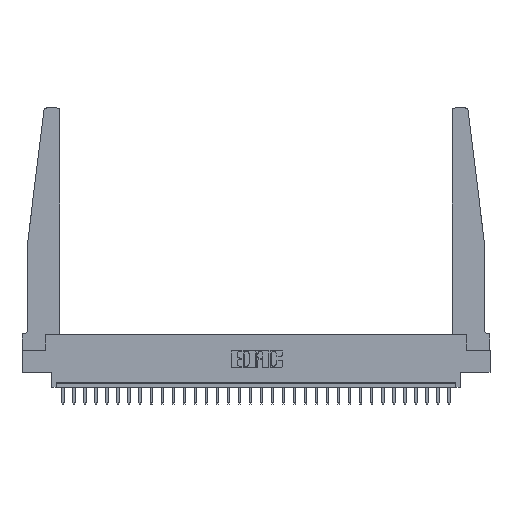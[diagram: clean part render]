
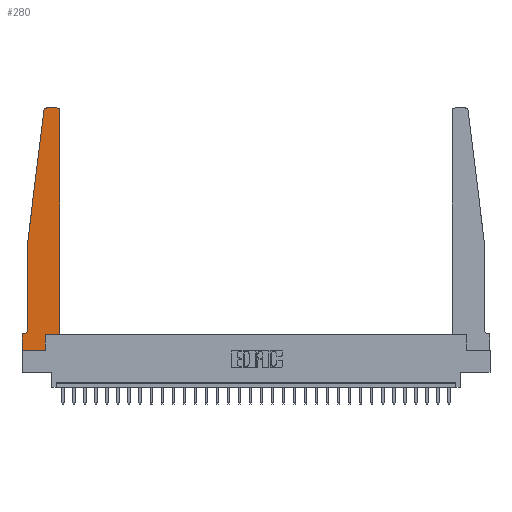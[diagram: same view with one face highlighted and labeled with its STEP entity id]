
A CAD part, top view. The second image highlights one B-rep face of the part: STEP entity #280.
In plain terms, the highlighted planar face has unit normal (0, 0, 1).
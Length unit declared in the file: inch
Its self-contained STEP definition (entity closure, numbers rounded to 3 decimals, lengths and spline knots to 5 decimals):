
#280 = ADVANCED_FACE ( 'NONE', ( #17258 ), #15068, .T. ) ;
#375 = CIRCLE ( 'NONE', #2223, 0.05 ) ;
#410 = VECTOR ( 'NONE', #20991, 39.37008 ) ;
#855 = CARTESIAN_POINT ( 'NONE',  ( 0.2605, 0.18, 0.37 ) ) ;
#1025 = DIRECTION ( 'NONE',  ( -1., 0., 0. ) ) ;
#1101 = EDGE_CURVE ( 'NONE', #24058, #24308, #16707, .T. ) ;
#1315 = CARTESIAN_POINT ( 'NONE',  ( 0., 0., 0.37 ) ) ;
#1605 = CARTESIAN_POINT ( 'NONE',  ( 0.395, 2.75, 0.37 ) ) ;
#1904 = CARTESIAN_POINT ( 'NONE',  ( 0., 0.1875, 0.37 ) ) ;
#2104 = EDGE_LOOP ( 'NONE', ( #17373, #17752, #11863, #24557, #27052, #9151, #11332, #17561, #2962, #5431, #9153, #21546 ) ) ;
#2171 = DIRECTION ( 'NONE',  ( 0., 0., 1. ) ) ;
#2223 = AXIS2_PLACEMENT_3D ( 'NONE', #21859, #21561, #15331 ) ;
#2415 = EDGE_CURVE ( 'NONE', #8377, #7073, #9239, .T. ) ;
#2419 = CARTESIAN_POINT ( 'NONE',  ( 0.2605, 0.18, 0.37 ) ) ;
#2713 = CARTESIAN_POINT ( 'NONE',  ( 0., 0., 0.37 ) ) ;
#2962 = ORIENTED_EDGE ( 'NONE', *, *, #15826, .T. ) ;
#3213 = VECTOR ( 'NONE', #13120, 39.37008 ) ;
#3463 = LINE ( 'NONE', #855, #19608 ) ;
#3505 = CARTESIAN_POINT ( 'NONE',  ( 0.2605, 0., 0.37 ) ) ;
#4042 = EDGE_CURVE ( 'NONE', #24308, #20543, #25350, .T. ) ;
#4122 = VERTEX_POINT ( 'NONE', #23754 ) ;
#4475 = LINE ( 'NONE', #24180, #3213 ) ;
#5311 = DIRECTION ( 'NONE',  ( 0., 1., 0. ) ) ;
#5431 = ORIENTED_EDGE ( 'NONE', *, *, #23795, .T. ) ;
#5452 = VECTOR ( 'NONE', #21392, 39.37008 ) ;
#5654 = AXIS2_PLACEMENT_3D ( 'NONE', #1904, #23916, #10833 ) ;
#5894 = EDGE_CURVE ( 'NONE', #11789, #4122, #375, .T. ) ;
#6534 = LINE ( 'NONE', #15383, #9674 ) ;
#7073 = VERTEX_POINT ( 'NONE', #15373 ) ;
#7841 = CARTESIAN_POINT ( 'NONE',  ( 0.425, 0.18, 0.37 ) ) ;
#8126 = DIRECTION ( 'NONE',  ( 1., 0., 0. ) ) ;
#8315 = VECTOR ( 'NONE', #11732, 39.37008 ) ;
#8377 = VERTEX_POINT ( 'NONE', #17723 ) ;
#8596 = VECTOR ( 'NONE', #1025, 39.37008 ) ;
#9109 = EDGE_CURVE ( 'NONE', #25172, #11789, #6534, .T. ) ;
#9151 = ORIENTED_EDGE ( 'NONE', *, *, #18477, .T. ) ;
#9153 = ORIENTED_EDGE ( 'NONE', *, *, #9848, .T. ) ;
#9239 = LINE ( 'NONE', #2713, #23352 ) ;
#9674 = VECTOR ( 'NONE', #24224, 39.37008 ) ;
#9848 = EDGE_CURVE ( 'NONE', #23096, #24058, #13945, .T. ) ;
#10488 = VERTEX_POINT ( 'NONE', #12768 ) ;
#10833 = DIRECTION ( 'NONE',  ( 1., 0., 0. ) ) ;
#11331 = DIRECTION ( 'NONE',  ( 0., 0., 1. ) ) ;
#11332 = ORIENTED_EDGE ( 'NONE', *, *, #2415, .T. ) ;
#11732 = DIRECTION ( 'NONE',  ( 0., 1., 0. ) ) ;
#11789 = VERTEX_POINT ( 'NONE', #21066 ) ;
#11863 = ORIENTED_EDGE ( 'NONE', *, *, #24391, .T. ) ;
#11987 = LINE ( 'NONE', #20853, #18716 ) ;
#12255 = CARTESIAN_POINT ( 'NONE',  ( 0.25, 2.75, 0.37 ) ) ;
#12768 = CARTESIAN_POINT ( 'NONE',  ( 0.24675, 2.72367, 0.37 ) ) ;
#13120 = DIRECTION ( 'NONE',  ( -0.122, -0.992, 0. ) ) ;
#13945 = LINE ( 'NONE', #25256, #8315 ) ;
#14062 = VERTEX_POINT ( 'NONE', #3505 ) ;
#14251 = CARTESIAN_POINT ( 'NONE',  ( 0.425, 2.72, 0.37 ) ) ;
#14354 = AXIS2_PLACEMENT_3D ( 'NONE', #19769, #11331, #17905 ) ;
#15068 = PLANE ( 'NONE',  #5654 ) ;
#15331 = DIRECTION ( 'NONE',  ( -1., 0., 0. ) ) ;
#15373 = CARTESIAN_POINT ( 'NONE',  ( 0., 0., 0.37 ) ) ;
#15383 = CARTESIAN_POINT ( 'NONE',  ( 0.065, 1.25, 0.37 ) ) ;
#15744 = CIRCLE ( 'NONE', #14354, 0.03 ) ;
#15826 = EDGE_CURVE ( 'NONE', #14062, #19433, #3463, .T. ) ;
#16707 = CIRCLE ( 'NONE', #27169, 0.03 ) ;
#17121 = CARTESIAN_POINT ( 'NONE',  ( 0.395, 2.72, 0.37 ) ) ;
#17197 = LINE ( 'NONE', #27630, #5452 ) ;
#17258 = FACE_OUTER_BOUND ( 'NONE', #2104, .T. ) ;
#17373 = ORIENTED_EDGE ( 'NONE', *, *, #4042, .T. ) ;
#17403 = DIRECTION ( 'NONE',  ( 0., -1., 0. ) ) ;
#17561 = ORIENTED_EDGE ( 'NONE', *, *, #22574, .T. ) ;
#17723 = CARTESIAN_POINT ( 'NONE',  ( 0., 0.1875, 0.37 ) ) ;
#17752 = ORIENTED_EDGE ( 'NONE', *, *, #26109, .T. ) ;
#17905 = DIRECTION ( 'NONE',  ( 1., 0., 0. ) ) ;
#18477 = EDGE_CURVE ( 'NONE', #4122, #8377, #11987, .T. ) ;
#18716 = VECTOR ( 'NONE', #25371, 39.37008 ) ;
#18942 = CARTESIAN_POINT ( 'NONE',  ( 0.27653, 2.75, 0.37 ) ) ;
#19433 = VERTEX_POINT ( 'NONE', #2419 ) ;
#19608 = VECTOR ( 'NONE', #5311, 39.37008 ) ;
#19769 = CARTESIAN_POINT ( 'NONE',  ( 0.27653, 2.72, 0.37 ) ) ;
#20543 = VERTEX_POINT ( 'NONE', #18942 ) ;
#20853 = CARTESIAN_POINT ( 'NONE',  ( 0.065, 0.1875, 0.37 ) ) ;
#20991 = DIRECTION ( 'NONE',  ( 1., 0., 0. ) ) ;
#21066 = CARTESIAN_POINT ( 'NONE',  ( 0.065, 0.2375, 0.37 ) ) ;
#21392 = DIRECTION ( 'NONE',  ( 1., 0., 0. ) ) ;
#21546 = ORIENTED_EDGE ( 'NONE', *, *, #1101, .T. ) ;
#21561 = DIRECTION ( 'NONE',  ( 0., 0., -1. ) ) ;
#21859 = CARTESIAN_POINT ( 'NONE',  ( 0.015, 0.2375, 0.37 ) ) ;
#21888 = CARTESIAN_POINT ( 'NONE',  ( 0.065, 1.25, 0.37 ) ) ;
#22574 = EDGE_CURVE ( 'NONE', #7073, #14062, #27821, .T. ) ;
#23096 = VERTEX_POINT ( 'NONE', #7841 ) ;
#23352 = VECTOR ( 'NONE', #17403, 39.37008 ) ;
#23754 = CARTESIAN_POINT ( 'NONE',  ( 0.015, 0.1875, 0.37 ) ) ;
#23795 = EDGE_CURVE ( 'NONE', #19433, #23096, #17197, .T. ) ;
#23916 = DIRECTION ( 'NONE',  ( 0., 0., 1. ) ) ;
#24058 = VERTEX_POINT ( 'NONE', #14251 ) ;
#24180 = CARTESIAN_POINT ( 'NONE',  ( 0.065, 1.25, 0.37 ) ) ;
#24224 = DIRECTION ( 'NONE',  ( 0., -1., 0. ) ) ;
#24308 = VERTEX_POINT ( 'NONE', #1605 ) ;
#24391 = EDGE_CURVE ( 'NONE', #10488, #25172, #4475, .T. ) ;
#24557 = ORIENTED_EDGE ( 'NONE', *, *, #9109, .T. ) ;
#25172 = VERTEX_POINT ( 'NONE', #21888 ) ;
#25256 = CARTESIAN_POINT ( 'NONE',  ( 0.425, 0.18, 0.37 ) ) ;
#25350 = LINE ( 'NONE', #12255, #8596 ) ;
#25371 = DIRECTION ( 'NONE',  ( -1., 0., 0. ) ) ;
#26109 = EDGE_CURVE ( 'NONE', #20543, #10488, #15744, .T. ) ;
#27052 = ORIENTED_EDGE ( 'NONE', *, *, #5894, .T. ) ;
#27169 = AXIS2_PLACEMENT_3D ( 'NONE', #17121, #2171, #8126 ) ;
#27630 = CARTESIAN_POINT ( 'NONE',  ( 0.425, 0.18, 0.37 ) ) ;
#27821 = LINE ( 'NONE', #1315, #410 ) ;
